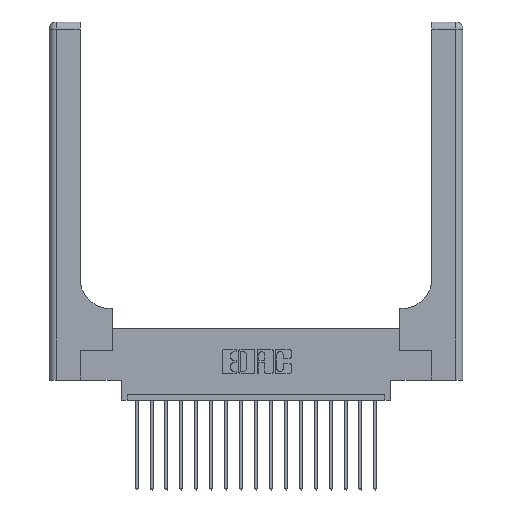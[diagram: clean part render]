
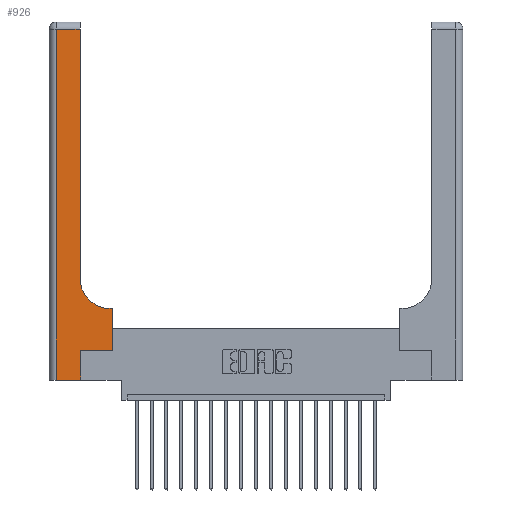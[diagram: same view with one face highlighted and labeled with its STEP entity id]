
A CAD part, top view. The second image highlights one B-rep face of the part: STEP entity #926.
In plain terms, the highlighted planar face has unit normal (0, 0, 1).
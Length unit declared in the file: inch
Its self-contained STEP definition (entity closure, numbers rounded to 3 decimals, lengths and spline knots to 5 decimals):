
#483 = ORIENTED_EDGE ( 'NONE', *, *, #11864, .T. ) ;
#502 = ORIENTED_EDGE ( 'NONE', *, *, #16851, .T. ) ;
#926 = ADVANCED_FACE ( 'NONE', ( #3509 ), #18589, .F. ) ;
#1552 = CARTESIAN_POINT ( 'NONE',  ( 0.528, 0.25, 0.37 ) ) ;
#2029 = CARTESIAN_POINT ( 'NONE',  ( 0.06, 0., 0.37 ) ) ;
#2356 = LINE ( 'NONE', #9925, #3987 ) ;
#2429 = CARTESIAN_POINT ( 'NONE',  ( 0.265, 0., 0.37 ) ) ;
#2572 = ORIENTED_EDGE ( 'NONE', *, *, #4839, .T. ) ;
#2604 = ORIENTED_EDGE ( 'NONE', *, *, #7242, .T. ) ;
#2721 = LINE ( 'NONE', #8561, #6204 ) ;
#3509 = FACE_OUTER_BOUND ( 'NONE', #15942, .T. ) ;
#3605 = LINE ( 'NONE', #19173, #4979 ) ;
#3813 = CIRCLE ( 'NONE', #14924, 0.25 ) ;
#3828 = CARTESIAN_POINT ( 'NONE',  ( 0.51, 0.85, 0.37 ) ) ;
#3983 = DIRECTION ( 'NONE',  ( 0., 1., 0. ) ) ;
#3987 = VECTOR ( 'NONE', #3983, 39.37008 ) ;
#4158 = VECTOR ( 'NONE', #17984, 39.37008 ) ;
#4578 = ORIENTED_EDGE ( 'NONE', *, *, #5759, .T. ) ;
#4673 = VERTEX_POINT ( 'NONE', #16816 ) ;
#4839 = EDGE_CURVE ( 'NONE', #15099, #15968, #3813, .T. ) ;
#4979 = VECTOR ( 'NONE', #10632, 39.37008 ) ;
#5731 = VECTOR ( 'NONE', #7409, 39.37008 ) ;
#5759 = EDGE_CURVE ( 'NONE', #11268, #14058, #8128, .T. ) ;
#5998 = CARTESIAN_POINT ( 'NONE',  ( 0.265, 0.25, 0.37 ) ) ;
#6043 = DIRECTION ( 'NONE',  ( 0., 1., 0. ) ) ;
#6204 = VECTOR ( 'NONE', #7090, 39.37008 ) ;
#6743 = DIRECTION ( 'NONE',  ( 1., 0., 0. ) ) ;
#7090 = DIRECTION ( 'NONE',  ( -1., 0., 0. ) ) ;
#7117 = AXIS2_PLACEMENT_3D ( 'NONE', #15597, #12701, #9678 ) ;
#7242 = EDGE_CURVE ( 'NONE', #15968, #13188, #9005, .T. ) ;
#7409 = DIRECTION ( 'NONE',  ( -1., 0., 0. ) ) ;
#7451 = VERTEX_POINT ( 'NONE', #7735 ) ;
#7735 = CARTESIAN_POINT ( 'NONE',  ( 0.528, 0.6, 0.37 ) ) ;
#8128 = LINE ( 'NONE', #17160, #13750 ) ;
#8425 = CARTESIAN_POINT ( 'NONE',  ( 0.26, 3., 0.37 ) ) ;
#8561 = CARTESIAN_POINT ( 'NONE',  ( 0.26, 0.6, 0.37 ) ) ;
#8824 = CARTESIAN_POINT ( 'NONE',  ( 0., 2.94, 0.37 ) ) ;
#9005 = LINE ( 'NONE', #8425, #4158 ) ;
#9667 = EDGE_CURVE ( 'NONE', #7451, #15099, #2721, .T. ) ;
#9678 = DIRECTION ( 'NONE',  ( -1., 0., 0. ) ) ;
#9715 = ORIENTED_EDGE ( 'NONE', *, *, #14914, .T. ) ;
#9925 = CARTESIAN_POINT ( 'NONE',  ( 0.265, 0., 0.37 ) ) ;
#9988 = ORIENTED_EDGE ( 'NONE', *, *, #9667, .T. ) ;
#10028 = ORIENTED_EDGE ( 'NONE', *, *, #12452, .T. ) ;
#10632 = DIRECTION ( 'NONE',  ( 0., -1., 0. ) ) ;
#11268 = VERTEX_POINT ( 'NONE', #2029 ) ;
#11577 = LINE ( 'NONE', #5998, #16491 ) ;
#11864 = EDGE_CURVE ( 'NONE', #15030, #11268, #3605, .T. ) ;
#12452 = EDGE_CURVE ( 'NONE', #14058, #4673, #2356, .T. ) ;
#12701 = DIRECTION ( 'NONE',  ( 0., 0., -1. ) ) ;
#12789 = CARTESIAN_POINT ( 'NONE',  ( 0.26, 0.85, 0.37 ) ) ;
#13061 = CARTESIAN_POINT ( 'NONE',  ( 0.528, 0.25, 0.37 ) ) ;
#13188 = VERTEX_POINT ( 'NONE', #18220 ) ;
#13750 = VECTOR ( 'NONE', #15515, 39.37008 ) ;
#14058 = VERTEX_POINT ( 'NONE', #2429 ) ;
#14156 = DIRECTION ( 'NONE',  ( 0., 0., -1. ) ) ;
#14278 = LINE ( 'NONE', #1552, #18025 ) ;
#14912 = ORIENTED_EDGE ( 'NONE', *, *, #14913, .T. ) ;
#14913 = EDGE_CURVE ( 'NONE', #4673, #18880, #11577, .T. ) ;
#14914 = EDGE_CURVE ( 'NONE', #13188, #15030, #18824, .T. ) ;
#14924 = AXIS2_PLACEMENT_3D ( 'NONE', #3828, #14156, #6743 ) ;
#15030 = VERTEX_POINT ( 'NONE', #15182 ) ;
#15099 = VERTEX_POINT ( 'NONE', #15379 ) ;
#15182 = CARTESIAN_POINT ( 'NONE',  ( 0.06, 2.94, 0.37 ) ) ;
#15379 = CARTESIAN_POINT ( 'NONE',  ( 0.51, 0.6, 0.37 ) ) ;
#15515 = DIRECTION ( 'NONE',  ( 1., 0., 0. ) ) ;
#15597 = CARTESIAN_POINT ( 'NONE',  ( 0., 3., 0.37 ) ) ;
#15942 = EDGE_LOOP ( 'NONE', ( #2604, #9715, #483, #4578, #10028, #14912, #502, #9988, #2572 ) ) ;
#15968 = VERTEX_POINT ( 'NONE', #12789 ) ;
#16491 = VECTOR ( 'NONE', #17982, 39.37008 ) ;
#16816 = CARTESIAN_POINT ( 'NONE',  ( 0.265, 0.25, 0.37 ) ) ;
#16851 = EDGE_CURVE ( 'NONE', #18880, #7451, #14278, .T. ) ;
#17160 = CARTESIAN_POINT ( 'NONE',  ( 0., 0., 0.37 ) ) ;
#17982 = DIRECTION ( 'NONE',  ( 1., 0., 0. ) ) ;
#17984 = DIRECTION ( 'NONE',  ( 0., 1., 0. ) ) ;
#18025 = VECTOR ( 'NONE', #6043, 39.37008 ) ;
#18220 = CARTESIAN_POINT ( 'NONE',  ( 0.26, 2.94, 0.37 ) ) ;
#18589 = PLANE ( 'NONE',  #7117 ) ;
#18824 = LINE ( 'NONE', #8824, #5731 ) ;
#18880 = VERTEX_POINT ( 'NONE', #13061 ) ;
#19173 = CARTESIAN_POINT ( 'NONE',  ( 0.06, 3., 0.37 ) ) ;
